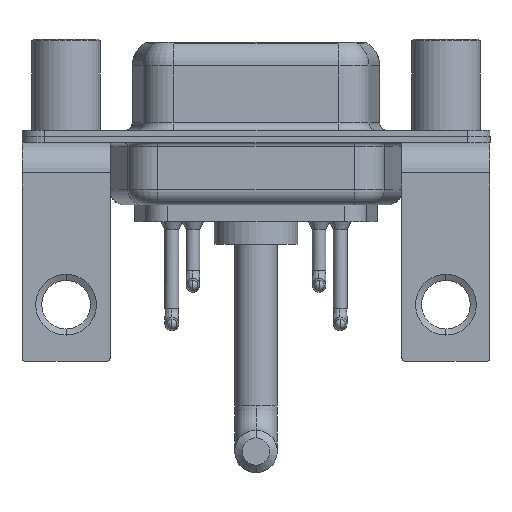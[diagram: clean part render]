
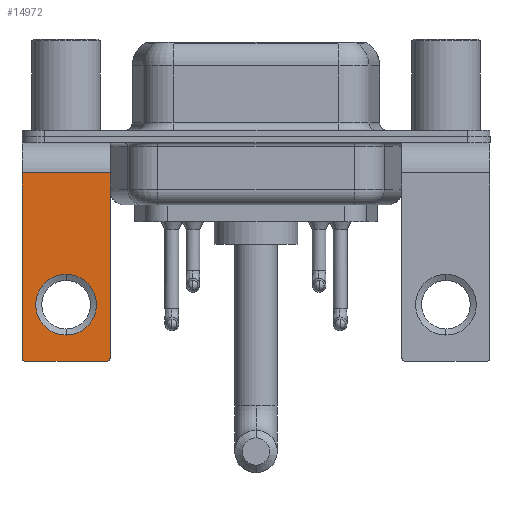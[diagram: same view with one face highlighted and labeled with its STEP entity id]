
A CAD part, front view. The second image highlights one B-rep face of the part: STEP entity #14972.
In plain terms, the highlighted planar face has unit normal (0, -1, 0).
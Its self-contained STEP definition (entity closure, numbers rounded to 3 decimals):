
#158 = ORIENTED_EDGE ( 'NONE', *, *, #11566, .T. ) ;
#203 = CARTESIAN_POINT ( 'NONE',  ( 0., -6.25, -13.07 ) ) ;
#264 = EDGE_CURVE ( 'NONE', #13432, #10006, #11734, .T. ) ;
#686 = CARTESIAN_POINT ( 'NONE',  ( -2.9, -6.25, -2.4 ) ) ;
#863 = CARTESIAN_POINT ( 'NONE',  ( 2.9, -6.25, -2.4 ) ) ;
#920 = EDGE_LOOP ( 'NONE', ( #7996, #15506 ) ) ;
#1454 = CARTESIAN_POINT ( 'NONE',  ( -2.65, -6.25, -14.8 ) ) ;
#1954 = CARTESIAN_POINT ( 'NONE',  ( 0., -6.25, -11.07 ) ) ;
#1995 = CARTESIAN_POINT ( 'NONE',  ( 2.65, -6.25, -14.55 ) ) ;
#2166 = VERTEX_POINT ( 'NONE', #2438 ) ;
#2213 = DIRECTION ( 'NONE',  ( 0., 1., 0. ) ) ;
#2438 = CARTESIAN_POINT ( 'NONE',  ( 0., -6.25, -9.07 ) ) ;
#2439 = ORIENTED_EDGE ( 'NONE', *, *, #18038, .F. ) ;
#2685 = VECTOR ( 'NONE', #11601, 1000. ) ;
#3615 = AXIS2_PLACEMENT_3D ( 'NONE', #7041, #11434, #12750 ) ;
#3908 = DIRECTION ( 'NONE',  ( 0., 0., 1. ) ) ;
#4105 = VECTOR ( 'NONE', #12472, 1000. ) ;
#4531 = AXIS2_PLACEMENT_3D ( 'NONE', #18648, #8478, #15256 ) ;
#4695 = VERTEX_POINT ( 'NONE', #1454 ) ;
#4901 = EDGE_CURVE ( 'NONE', #14674, #13240, #18098, .T. ) ;
#4902 = CIRCLE ( 'NONE', #11010, 2. ) ;
#4947 = EDGE_CURVE ( 'NONE', #2166, #11705, #4902, .T. ) ;
#5060 = FACE_BOUND ( 'NONE', #920, .T. ) ;
#5215 = EDGE_LOOP ( 'NONE', ( #5920, #18782, #2439, #7680, #13604, #158 ) ) ;
#5920 = ORIENTED_EDGE ( 'NONE', *, *, #4901, .T. ) ;
#6249 = EDGE_CURVE ( 'NONE', #11705, #2166, #8565, .T. ) ;
#6288 = CARTESIAN_POINT ( 'NONE',  ( 2.65, -6.25, -14.8 ) ) ;
#6636 = CIRCLE ( 'NONE', #3615, 0.25 ) ;
#7041 = CARTESIAN_POINT ( 'NONE',  ( -2.65, -6.25, -14.55 ) ) ;
#7680 = ORIENTED_EDGE ( 'NONE', *, *, #264, .T. ) ;
#7803 = DIRECTION ( 'NONE',  ( 0., 0., 1. ) ) ;
#7996 = ORIENTED_EDGE ( 'NONE', *, *, #6249, .T. ) ;
#8478 = DIRECTION ( 'NONE',  ( 0., 1., 0. ) ) ;
#8565 = CIRCLE ( 'NONE', #9164, 2. ) ;
#8982 = VECTOR ( 'NONE', #12317, 1000. ) ;
#9164 = AXIS2_PLACEMENT_3D ( 'NONE', #1954, #10808, #13654 ) ;
#9351 = CARTESIAN_POINT ( 'NONE',  ( 2.9, -6.25, -2.4 ) ) ;
#9537 = CARTESIAN_POINT ( 'NONE',  ( 2.9, -6.25, -14.55 ) ) ;
#10006 = VERTEX_POINT ( 'NONE', #9537 ) ;
#10443 = CARTESIAN_POINT ( 'NONE',  ( 2.9, -6.25, -2.4 ) ) ;
#10808 = DIRECTION ( 'NONE',  ( 0., 1., 0. ) ) ;
#11010 = AXIS2_PLACEMENT_3D ( 'NONE', #16780, #2213, #3908 ) ;
#11216 = LINE ( 'NONE', #11309, #2685 ) ;
#11309 = CARTESIAN_POINT ( 'NONE',  ( 2.9, -6.25, -14.8 ) ) ;
#11434 = DIRECTION ( 'NONE',  ( 0., -1., 0. ) ) ;
#11566 = EDGE_CURVE ( 'NONE', #16004, #14674, #12226, .T. ) ;
#11601 = DIRECTION ( 'NONE',  ( -1., 0., 0. ) ) ;
#11705 = VERTEX_POINT ( 'NONE', #203 ) ;
#11734 = CIRCLE ( 'NONE', #12931, 0.25 ) ;
#12016 = EDGE_CURVE ( 'NONE', #16004, #10006, #15321, .T. ) ;
#12025 = CARTESIAN_POINT ( 'NONE',  ( -2.9, -6.25, -14.55 ) ) ;
#12226 = LINE ( 'NONE', #9351, #8982 ) ;
#12317 = DIRECTION ( 'NONE',  ( -1., 0., 0. ) ) ;
#12398 = DIRECTION ( 'NONE',  ( 0., 0., -1. ) ) ;
#12472 = DIRECTION ( 'NONE',  ( 0., 0., -1. ) ) ;
#12750 = DIRECTION ( 'NONE',  ( 0., 0., 1. ) ) ;
#12931 = AXIS2_PLACEMENT_3D ( 'NONE', #1995, #18165, #7803 ) ;
#13240 = VERTEX_POINT ( 'NONE', #12025 ) ;
#13432 = VERTEX_POINT ( 'NONE', #6288 ) ;
#13604 = ORIENTED_EDGE ( 'NONE', *, *, #12016, .F. ) ;
#13654 = DIRECTION ( 'NONE',  ( 0., 0., 1. ) ) ;
#14179 = FACE_OUTER_BOUND ( 'NONE', #5215, .T. ) ;
#14674 = VERTEX_POINT ( 'NONE', #14700 ) ;
#14700 = CARTESIAN_POINT ( 'NONE',  ( -2.9, -6.25, -2.4 ) ) ;
#14920 = EDGE_CURVE ( 'NONE', #13240, #4695, #6636, .T. ) ;
#14972 = ADVANCED_FACE ( 'NONE', ( #5060, #14179 ), #17139, .F. ) ;
#15256 = DIRECTION ( 'NONE',  ( 0., 0., 1. ) ) ;
#15321 = LINE ( 'NONE', #863, #4105 ) ;
#15506 = ORIENTED_EDGE ( 'NONE', *, *, #4947, .T. ) ;
#16004 = VERTEX_POINT ( 'NONE', #10443 ) ;
#16493 = VECTOR ( 'NONE', #12398, 1000. ) ;
#16780 = CARTESIAN_POINT ( 'NONE',  ( 0., -6.25, -11.07 ) ) ;
#17139 = PLANE ( 'NONE',  #4531 ) ;
#18038 = EDGE_CURVE ( 'NONE', #13432, #4695, #11216, .T. ) ;
#18098 = LINE ( 'NONE', #686, #16493 ) ;
#18165 = DIRECTION ( 'NONE',  ( 0., -1., 0. ) ) ;
#18648 = CARTESIAN_POINT ( 'NONE',  ( 2.9, -6.25, -2.4 ) ) ;
#18782 = ORIENTED_EDGE ( 'NONE', *, *, #14920, .T. ) ;
